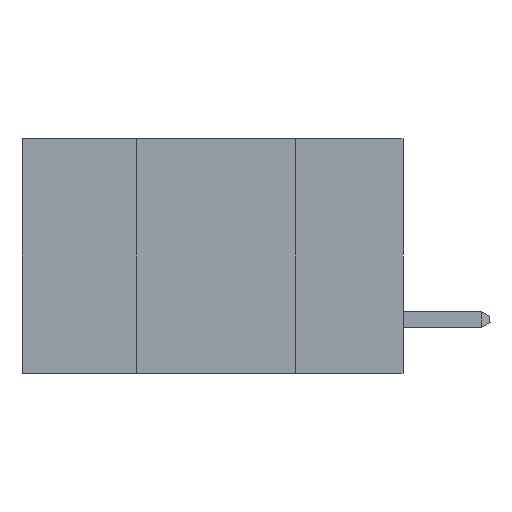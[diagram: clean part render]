
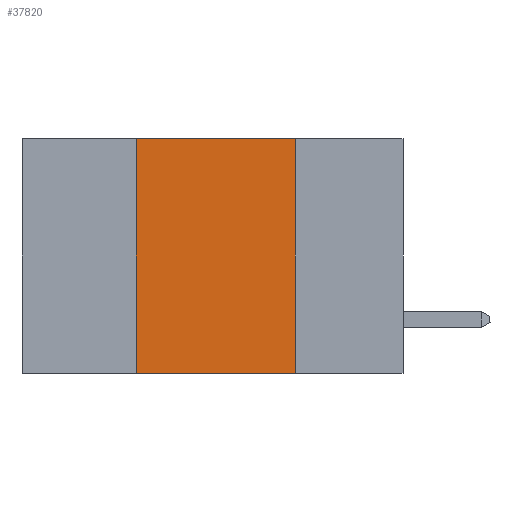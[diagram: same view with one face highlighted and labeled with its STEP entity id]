
A CAD part, left-side view. The second image highlights one B-rep face of the part: STEP entity #37820.
In plain terms, the highlighted planar face has unit normal (-1, 0, 0).
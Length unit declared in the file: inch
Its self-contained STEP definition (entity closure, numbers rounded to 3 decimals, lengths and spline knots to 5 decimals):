
#3011 = DIRECTION ( 'NONE',  ( 0., 0., -1. ) ) ;
#3522 = ORIENTED_EDGE ( 'NONE', *, *, #17750, .F. ) ;
#5770 = VECTOR ( 'NONE', #6133, 39.37008 ) ;
#5999 = VECTOR ( 'NONE', #16594, 39.37008 ) ;
#6121 = CARTESIAN_POINT ( 'NONE',  ( 0., 0.6, -0.37 ) ) ;
#6133 = DIRECTION ( 'NONE',  ( 0., 0., -1. ) ) ;
#6788 = CARTESIAN_POINT ( 'NONE',  ( 0., 0.17, 0. ) ) ;
#9837 = VERTEX_POINT ( 'NONE', #24725 ) ;
#13551 = VERTEX_POINT ( 'NONE', #38380 ) ;
#13800 = CARTESIAN_POINT ( 'NONE',  ( 0., 0.17, 0. ) ) ;
#14146 = DIRECTION ( 'NONE',  ( 1., 0., 0. ) ) ;
#16108 = DIRECTION ( 'NONE',  ( 0., -1., 0. ) ) ;
#16594 = DIRECTION ( 'NONE',  ( 0., -1., 0. ) ) ;
#17721 = LINE ( 'NONE', #48128, #36403 ) ;
#17750 = EDGE_CURVE ( 'NONE', #27333, #9837, #30369, .T. ) ;
#20664 = VERTEX_POINT ( 'NONE', #28081 ) ;
#23844 = ORIENTED_EDGE ( 'NONE', *, *, #29289, .F. ) ;
#24725 = CARTESIAN_POINT ( 'NONE',  ( 0., 0.17, -0.37 ) ) ;
#27092 = CARTESIAN_POINT ( 'NONE',  ( 0., 0.6, 0. ) ) ;
#27333 = VERTEX_POINT ( 'NONE', #13800 ) ;
#27594 = AXIS2_PLACEMENT_3D ( 'NONE', #43777, #14146, #3011 ) ;
#28081 = CARTESIAN_POINT ( 'NONE',  ( 0., 0.42, -0.37 ) ) ;
#29289 = EDGE_CURVE ( 'NONE', #20664, #13551, #17721, .T. ) ;
#29386 = LINE ( 'NONE', #27092, #33419 ) ;
#30369 = LINE ( 'NONE', #6788, #5770 ) ;
#31063 = ORIENTED_EDGE ( 'NONE', *, *, #43197, .F. ) ;
#33419 = VECTOR ( 'NONE', #16108, 39.37008 ) ;
#36403 = VECTOR ( 'NONE', #37034, 39.37008 ) ;
#37034 = DIRECTION ( 'NONE',  ( 0., 0., 1. ) ) ;
#37820 = ADVANCED_FACE ( 'NONE', ( #47166 ), #47870, .F. ) ;
#38380 = CARTESIAN_POINT ( 'NONE',  ( 0., 0.42, 0. ) ) ;
#40098 = EDGE_CURVE ( 'NONE', #20664, #9837, #42741, .T. ) ;
#42741 = LINE ( 'NONE', #6121, #5999 ) ;
#43197 = EDGE_CURVE ( 'NONE', #13551, #27333, #29386, .T. ) ;
#43362 = EDGE_LOOP ( 'NONE', ( #3522, #31063, #23844, #44474 ) ) ;
#43777 = CARTESIAN_POINT ( 'NONE',  ( 0., 0.6, 0. ) ) ;
#44474 = ORIENTED_EDGE ( 'NONE', *, *, #40098, .T. ) ;
#47166 = FACE_OUTER_BOUND ( 'NONE', #43362, .T. ) ;
#47870 = PLANE ( 'NONE',  #27594 ) ;
#48128 = CARTESIAN_POINT ( 'NONE',  ( 0., 0.42, 0. ) ) ;
